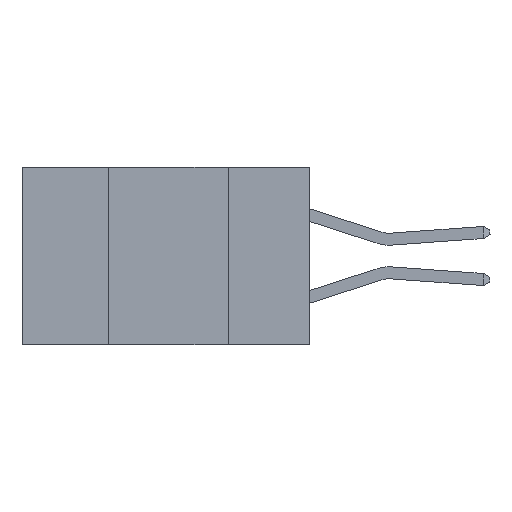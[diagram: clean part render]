
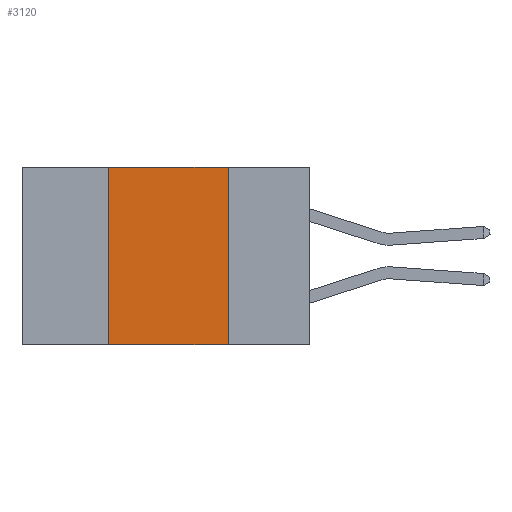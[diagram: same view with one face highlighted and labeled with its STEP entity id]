
A CAD part, left-side view. The second image highlights one B-rep face of the part: STEP entity #3120.
In plain terms, the highlighted planar face has unit normal (-1, 0, 0).
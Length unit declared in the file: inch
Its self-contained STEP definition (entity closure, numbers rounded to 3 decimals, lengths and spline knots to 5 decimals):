
#1231 = CARTESIAN_POINT ( 'NONE',  ( 0., 0.17, 0. ) ) ;
#2271 = DIRECTION ( 'NONE',  ( 1., 0., 0. ) ) ;
#3120 = ADVANCED_FACE ( 'NONE', ( #24592 ), #22496, .F. ) ;
#3430 = EDGE_CURVE ( 'NONE', #14779, #22463, #8038, .T. ) ;
#3773 = VECTOR ( 'NONE', #17917, 39.37008 ) ;
#5654 = LINE ( 'NONE', #8157, #23938 ) ;
#5793 = CARTESIAN_POINT ( 'NONE',  ( 0., 0.42, -0.37 ) ) ;
#6644 = DIRECTION ( 'NONE',  ( 0., 0., -1. ) ) ;
#8038 = LINE ( 'NONE', #8289, #26022 ) ;
#8157 = CARTESIAN_POINT ( 'NONE',  ( 0., 0.17, -0.37 ) ) ;
#8289 = CARTESIAN_POINT ( 'NONE',  ( 0., 0.6, 0. ) ) ;
#9558 = ORIENTED_EDGE ( 'NONE', *, *, #3430, .F. ) ;
#11045 = CARTESIAN_POINT ( 'NONE',  ( 0., 0.6, -0.37 ) ) ;
#12011 = EDGE_CURVE ( 'NONE', #25213, #14779, #26147, .T. ) ;
#13648 = AXIS2_PLACEMENT_3D ( 'NONE', #24718, #2271, #6644 ) ;
#14163 = EDGE_LOOP ( 'NONE', ( #15034, #9558, #25932, #24813 ) ) ;
#14779 = VERTEX_POINT ( 'NONE', #22693 ) ;
#15034 = ORIENTED_EDGE ( 'NONE', *, *, #24920, .F. ) ;
#15423 = LINE ( 'NONE', #11045, #23021 ) ;
#16183 = EDGE_CURVE ( 'NONE', #25213, #18057, #15423, .T. ) ;
#17917 = DIRECTION ( 'NONE',  ( 0., 0., 1. ) ) ;
#18057 = VERTEX_POINT ( 'NONE', #25624 ) ;
#19158 = DIRECTION ( 'NONE',  ( 0., -1., 0. ) ) ;
#22463 = VERTEX_POINT ( 'NONE', #1231 ) ;
#22496 = PLANE ( 'NONE',  #13648 ) ;
#22547 = DIRECTION ( 'NONE',  ( 0., -1., 0. ) ) ;
#22693 = CARTESIAN_POINT ( 'NONE',  ( 0., 0.42, 0. ) ) ;
#23021 = VECTOR ( 'NONE', #19158, 39.37008 ) ;
#23597 = CARTESIAN_POINT ( 'NONE',  ( 0., 0.42, -0.37 ) ) ;
#23938 = VECTOR ( 'NONE', #24385, 39.37008 ) ;
#24385 = DIRECTION ( 'NONE',  ( 0., 0., -1. ) ) ;
#24592 = FACE_OUTER_BOUND ( 'NONE', #14163, .T. ) ;
#24718 = CARTESIAN_POINT ( 'NONE',  ( 0., 0.6, 0. ) ) ;
#24813 = ORIENTED_EDGE ( 'NONE', *, *, #16183, .T. ) ;
#24920 = EDGE_CURVE ( 'NONE', #22463, #18057, #5654, .T. ) ;
#25213 = VERTEX_POINT ( 'NONE', #23597 ) ;
#25624 = CARTESIAN_POINT ( 'NONE',  ( 0., 0.17, -0.37 ) ) ;
#25932 = ORIENTED_EDGE ( 'NONE', *, *, #12011, .F. ) ;
#26022 = VECTOR ( 'NONE', #22547, 39.37008 ) ;
#26147 = LINE ( 'NONE', #5793, #3773 ) ;
